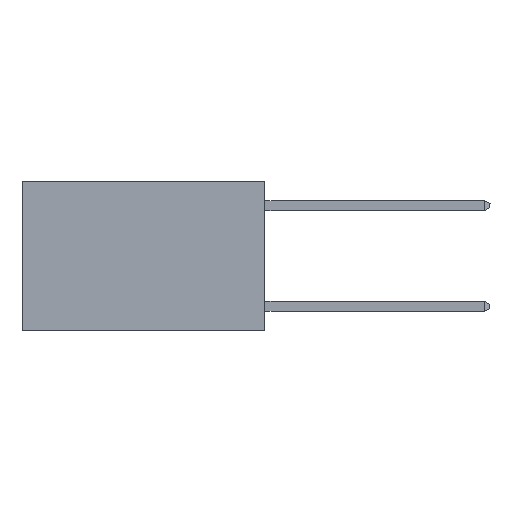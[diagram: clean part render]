
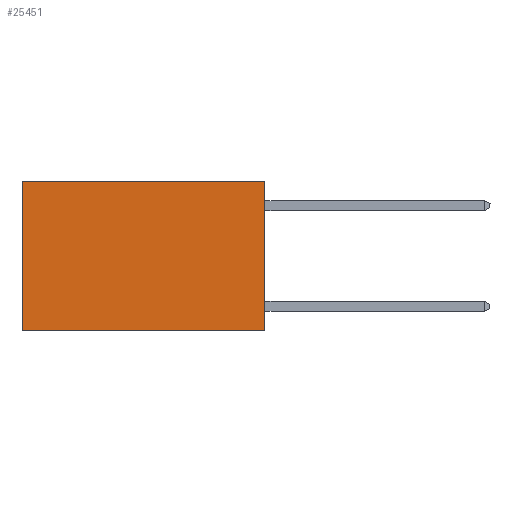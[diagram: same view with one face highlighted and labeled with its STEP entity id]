
A CAD part, left-side view. The second image highlights one B-rep face of the part: STEP entity #25451.
In plain terms, the highlighted planar face has unit normal (-1, 0, 0).
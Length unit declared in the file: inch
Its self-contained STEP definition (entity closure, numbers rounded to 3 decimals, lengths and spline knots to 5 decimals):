
#1002 = CARTESIAN_POINT ( 'NONE',  ( 0.2625, 0., 0. ) ) ;
#1099 = DIRECTION ( 'NONE',  ( 0., 1., 0. ) ) ;
#1157 = VECTOR ( 'NONE', #28604, 39.37008 ) ;
#2233 = EDGE_CURVE ( 'NONE', #7482, #26476, #18623, .T. ) ;
#3799 = VERTEX_POINT ( 'NONE', #14369 ) ;
#4709 = ORIENTED_EDGE ( 'NONE', *, *, #2233, .T. ) ;
#5136 = FACE_OUTER_BOUND ( 'NONE', #11546, .T. ) ;
#6817 = EDGE_CURVE ( 'NONE', #3799, #7482, #17585, .T. ) ;
#7101 = CARTESIAN_POINT ( 'NONE',  ( 0.2625, 0., -0.37 ) ) ;
#7482 = VERTEX_POINT ( 'NONE', #19370 ) ;
#11546 = EDGE_LOOP ( 'NONE', ( #4709, #20942, #22568, #18544 ) ) ;
#12369 = VECTOR ( 'NONE', #1099, 39.37008 ) ;
#12906 = DIRECTION ( 'NONE',  ( 0., 1., 0. ) ) ;
#13060 = EDGE_CURVE ( 'NONE', #3799, #15706, #21805, .T. ) ;
#14344 = PLANE ( 'NONE',  #24414 ) ;
#14369 = CARTESIAN_POINT ( 'NONE',  ( 0.2625, 0., 0. ) ) ;
#14829 = CARTESIAN_POINT ( 'NONE',  ( 0.2625, 0., -0.37 ) ) ;
#15706 = VERTEX_POINT ( 'NONE', #7101 ) ;
#16354 = DIRECTION ( 'NONE',  ( 0., 0., -1. ) ) ;
#17585 = LINE ( 'NONE', #19992, #21350 ) ;
#18544 = ORIENTED_EDGE ( 'NONE', *, *, #6817, .T. ) ;
#18623 = LINE ( 'NONE', #27827, #28436 ) ;
#19151 = CARTESIAN_POINT ( 'NONE',  ( 0.2625, 0., 0. ) ) ;
#19370 = CARTESIAN_POINT ( 'NONE',  ( 0.2625, 0.6, 0. ) ) ;
#19992 = CARTESIAN_POINT ( 'NONE',  ( 0.2625, 0., 0. ) ) ;
#20942 = ORIENTED_EDGE ( 'NONE', *, *, #24991, .F. ) ;
#21350 = VECTOR ( 'NONE', #12906, 39.37008 ) ;
#21805 = LINE ( 'NONE', #1002, #1157 ) ;
#22568 = ORIENTED_EDGE ( 'NONE', *, *, #13060, .F. ) ;
#24200 = CARTESIAN_POINT ( 'NONE',  ( 0.2625, 0.6, -0.37 ) ) ;
#24414 = AXIS2_PLACEMENT_3D ( 'NONE', #19151, #28354, #26082 ) ;
#24991 = EDGE_CURVE ( 'NONE', #15706, #26476, #26576, .T. ) ;
#25451 = ADVANCED_FACE ( 'NONE', ( #5136 ), #14344, .F. ) ;
#26082 = DIRECTION ( 'NONE',  ( 0., 0., -1. ) ) ;
#26476 = VERTEX_POINT ( 'NONE', #24200 ) ;
#26576 = LINE ( 'NONE', #14829, #12369 ) ;
#27827 = CARTESIAN_POINT ( 'NONE',  ( 0.2625, 0.6, 0. ) ) ;
#28354 = DIRECTION ( 'NONE',  ( 1., 0., 0. ) ) ;
#28436 = VECTOR ( 'NONE', #16354, 39.37008 ) ;
#28604 = DIRECTION ( 'NONE',  ( 0., 0., -1. ) ) ;
